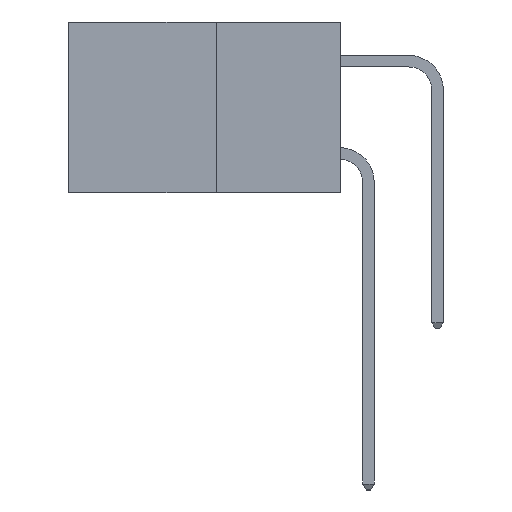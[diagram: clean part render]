
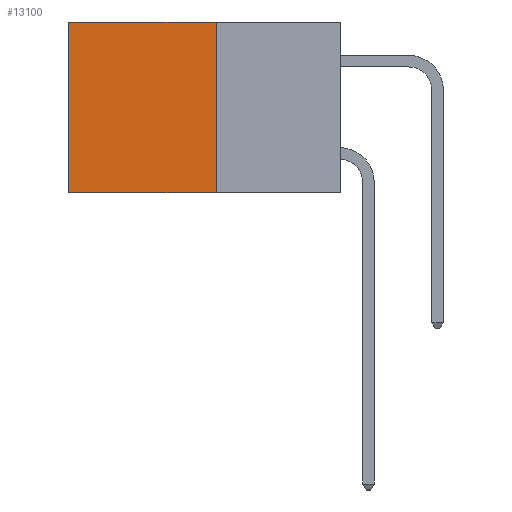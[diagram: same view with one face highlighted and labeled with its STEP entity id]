
A CAD part, left-side view. The second image highlights one B-rep face of the part: STEP entity #13100.
In plain terms, the highlighted planar face has unit normal (-1, 0, 0).
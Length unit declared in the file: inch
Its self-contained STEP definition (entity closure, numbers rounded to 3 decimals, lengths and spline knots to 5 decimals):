
#624 = CARTESIAN_POINT ( 'NONE',  ( 0.277, 0.27, -0.37 ) ) ;
#1206 = DIRECTION ( 'NONE',  ( 1., 0., 0. ) ) ;
#1944 = CARTESIAN_POINT ( 'NONE',  ( 0.277, 0.59, -0.37 ) ) ;
#1983 = DIRECTION ( 'NONE',  ( 0., 0., -1. ) ) ;
#2080 = CARTESIAN_POINT ( 'NONE',  ( 0.277, 0.59, -0.37 ) ) ;
#3101 = VECTOR ( 'NONE', #1983, 39.37008 ) ;
#3369 = VERTEX_POINT ( 'NONE', #6318 ) ;
#3449 = LINE ( 'NONE', #624, #6729 ) ;
#3994 = EDGE_CURVE ( 'NONE', #13094, #8453, #12448, .T. ) ;
#5239 = EDGE_CURVE ( 'NONE', #5541, #8453, #9694, .T. ) ;
#5541 = VERTEX_POINT ( 'NONE', #13173 ) ;
#5863 = CARTESIAN_POINT ( 'NONE',  ( 0.277, 0.27, 0. ) ) ;
#6318 = CARTESIAN_POINT ( 'NONE',  ( 0.277, 0.27, 0. ) ) ;
#6729 = VECTOR ( 'NONE', #8153, 39.37008 ) ;
#7632 = EDGE_CURVE ( 'NONE', #3369, #13094, #3449, .T. ) ;
#8153 = DIRECTION ( 'NONE',  ( 0., 0., -1. ) ) ;
#8453 = VERTEX_POINT ( 'NONE', #2080 ) ;
#8679 = EDGE_LOOP ( 'NONE', ( #13568, #12998, #12618, #12718 ) ) ;
#8685 = CARTESIAN_POINT ( 'NONE',  ( 0.277, 0.27, -0.37 ) ) ;
#9159 = VECTOR ( 'NONE', #13842, 39.37008 ) ;
#9694 = LINE ( 'NONE', #1944, #3101 ) ;
#9743 = EDGE_CURVE ( 'NONE', #3369, #5541, #15092, .T. ) ;
#9980 = DIRECTION ( 'NONE',  ( 0., 0., -1. ) ) ;
#11275 = CARTESIAN_POINT ( 'NONE',  ( 0.277, 0.27, -0.37 ) ) ;
#12448 = LINE ( 'NONE', #11275, #9159 ) ;
#12456 = FACE_OUTER_BOUND ( 'NONE', #8679, .T. ) ;
#12618 = ORIENTED_EDGE ( 'NONE', *, *, #7632, .F. ) ;
#12718 = ORIENTED_EDGE ( 'NONE', *, *, #9743, .T. ) ;
#12998 = ORIENTED_EDGE ( 'NONE', *, *, #3994, .F. ) ;
#13094 = VERTEX_POINT ( 'NONE', #13648 ) ;
#13100 = ADVANCED_FACE ( 'NONE', ( #12456 ), #14868, .F. ) ;
#13173 = CARTESIAN_POINT ( 'NONE',  ( 0.277, 0.59, 0. ) ) ;
#13568 = ORIENTED_EDGE ( 'NONE', *, *, #5239, .T. ) ;
#13648 = CARTESIAN_POINT ( 'NONE',  ( 0.277, 0.27, -0.37 ) ) ;
#13842 = DIRECTION ( 'NONE',  ( 0., 1., 0. ) ) ;
#14751 = VECTOR ( 'NONE', #15599, 39.37008 ) ;
#14868 = PLANE ( 'NONE',  #14878 ) ;
#14878 = AXIS2_PLACEMENT_3D ( 'NONE', #8685, #1206, #9980 ) ;
#15092 = LINE ( 'NONE', #5863, #14751 ) ;
#15599 = DIRECTION ( 'NONE',  ( 0., 1., 0. ) ) ;
